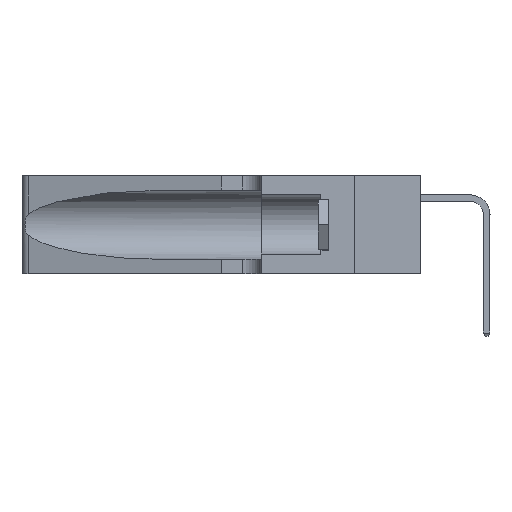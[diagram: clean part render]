
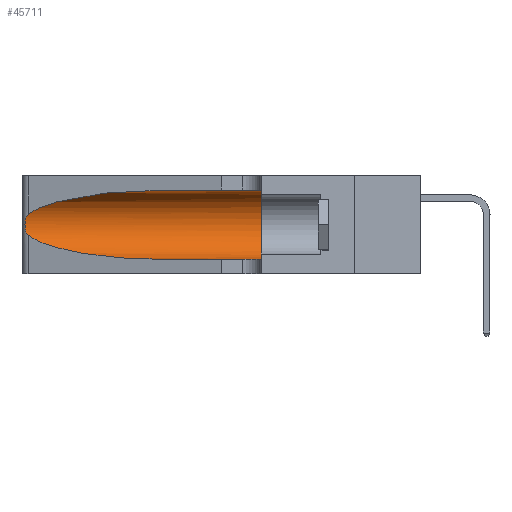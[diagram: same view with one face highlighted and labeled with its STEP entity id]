
A CAD part, left-side view. The second image highlights one B-rep face of the part: STEP entity #45711.
In plain terms, the highlighted cylindrical face has radius 3.308 mm (diameter 6.617 mm), a partial arc.
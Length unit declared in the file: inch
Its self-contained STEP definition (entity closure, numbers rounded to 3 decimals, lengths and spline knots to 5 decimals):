
#307 = DIRECTION ( 'NONE',  ( 0., 0., -1. ) ) ;
#678 = CARTESIAN_POINT ( 'NONE',  ( 0.25789, 1.23486, 0.15765 ) ) ;
#882 = EDGE_CURVE ( 'NONE', #23409, #2282, #24802, .T. ) ;
#1364 = VERTEX_POINT ( 'NONE', #19100 ) ;
#1776 =( BOUNDED_CURVE ( )  B_SPLINE_CURVE ( 3, ( #38948, #4856, #16434, #42914 ),
 .UNSPECIFIED., .F., .F. ) 
 B_SPLINE_CURVE_WITH_KNOTS ( ( 4, 4 ),
 ( 1.5708, 2.84003 ),
 .UNSPECIFIED. ) 
 CURVE ( )  GEOMETRIC_REPRESENTATION_ITEM ( )  RATIONAL_B_SPLINE_CURVE ( ( 1., 0.87, 0.87, 1. ) ) 
 REPRESENTATION_ITEM ( '' )  );
#2228 = CARTESIAN_POINT ( 'NONE',  ( 0.25487, 1.22718, 0.14631 ) ) ;
#2282 = VERTEX_POINT ( 'NONE', #2228 ) ;
#2468 = CARTESIAN_POINT ( 'NONE',  ( 0.1305, 0.72297, 0.05475 ) ) ;
#3626 = EDGE_CURVE ( 'NONE', #2282, #36121, #33569, .T. ) ;
#4567 = CARTESIAN_POINT ( 'NONE',  ( 0.25555, 1.22993, 0.14849 ) ) ;
#4856 = CARTESIAN_POINT ( 'NONE',  ( 0.18966, 0.96281, 0.31525 ) ) ;
#5522 = DIRECTION ( 'NONE',  ( 0., 1., 0. ) ) ;
#7322 = LINE ( 'NONE', #32075, #45301 ) ;
#7620 = EDGE_LOOP ( 'NONE', ( #49244, #40331, #35608, #29125, #20282, #24441 ) ) ;
#8314 = CARTESIAN_POINT ( 'NONE',  ( 0.25639, 1.23184, 0.21858 ) ) ;
#9125 = CYLINDRICAL_SURFACE ( 'NONE', #21257, 0.13025 ) ;
#9992 = EDGE_CURVE ( 'NONE', #36121, #33123, #7322, .T. ) ;
#12195 = CARTESIAN_POINT ( 'NONE',  ( 0.25787, 1.23484, 0.2124 ) ) ;
#14145 = VERTEX_POINT ( 'NONE', #47526 ) ;
#16002 = CARTESIAN_POINT ( 'NONE',  ( 0.26018, 1.23835, 0.19895 ) ) ;
#16434 = CARTESIAN_POINT ( 'NONE',  ( 0.2373, 1.15595, 0.28018 ) ) ;
#17002 = DIRECTION ( 'NONE',  ( 0., -1., 0. ) ) ;
#17243 = CARTESIAN_POINT ( 'NONE',  ( 0.1305, 0.72297, 0.05475 ) ) ;
#17751 = CARTESIAN_POINT ( 'NONE',  ( 0.2373, 1.15595, 0.08982 ) ) ;
#17806 = EDGE_CURVE ( 'NONE', #14145, #23409, #1776, .T. ) ;
#19100 = CARTESIAN_POINT ( 'NONE',  ( 0.1305, 0.35, 0.31525 ) ) ;
#19463 = CARTESIAN_POINT ( 'NONE',  ( 0.1305, 1.61858, 0.185 ) ) ;
#19827 = CARTESIAN_POINT ( 'NONE',  ( 0.26075, 1.23896, 0.178 ) ) ;
#20282 = ORIENTED_EDGE ( 'NONE', *, *, #33755, .F. ) ;
#20461 = FACE_OUTER_BOUND ( 'NONE', #7620, .T. ) ;
#21257 = AXIS2_PLACEMENT_3D ( 'NONE', #19463, #27067, #307 ) ;
#21596 = VECTOR ( 'NONE', #22932, 39.37008 ) ;
#22244 = CARTESIAN_POINT ( 'NONE',  ( 0.25487, 1.22718, 0.22369 ) ) ;
#22932 = DIRECTION ( 'NONE',  ( 0., -1., 0. ) ) ;
#23409 = VERTEX_POINT ( 'NONE', #22244 ) ;
#23631 = CARTESIAN_POINT ( 'NONE',  ( 0.25856, 1.23593, 0.16098 ) ) ;
#24441 = ORIENTED_EDGE ( 'NONE', *, *, #35800, .F. ) ;
#24802 = B_SPLINE_CURVE_WITH_KNOTS ( 'NONE', 3,
 ( #34852, #31068, #8314, #12195, #38648, #16002, #42487, #19827, #46276, #23631, #678, #27421, #4567, #31230 ),
 .UNSPECIFIED., .F., .F.,
 ( 4, 2, 2, 2, 2, 2, 4 ),
 ( 0., 0.00027, 0.00053, 0.00107, 0.0016, 0.00187, 0.00214 ),
 .UNSPECIFIED. ) ;
#25386 = CARTESIAN_POINT ( 'NONE',  ( 0.18966, 0.96281, 0.05475 ) ) ;
#27067 = DIRECTION ( 'NONE',  ( 0., -1., 0. ) ) ;
#27421 = CARTESIAN_POINT ( 'NONE',  ( 0.25639, 1.23186, 0.15144 ) ) ;
#28319 = CARTESIAN_POINT ( 'NONE',  ( 0.1305, 0.35, 0.185 ) ) ;
#29125 = ORIENTED_EDGE ( 'NONE', *, *, #9992, .T. ) ;
#31068 = CARTESIAN_POINT ( 'NONE',  ( 0.25555, 1.22994, 0.2215 ) ) ;
#31230 = CARTESIAN_POINT ( 'NONE',  ( 0.25487, 1.22718, 0.14631 ) ) ;
#32075 = CARTESIAN_POINT ( 'NONE',  ( 0.1305, 1.61858, 0.05475 ) ) ;
#32135 = DIRECTION ( 'NONE',  ( 0., 0., 1. ) ) ;
#32351 = CARTESIAN_POINT ( 'NONE',  ( 0.1305, 0.35, 0.05475 ) ) ;
#33123 = VERTEX_POINT ( 'NONE', #32351 ) ;
#33569 =( BOUNDED_CURVE ( )  B_SPLINE_CURVE ( 3, ( #44232, #17751, #25386, #2468 ),
 .UNSPECIFIED., .F., .T. ) 
 B_SPLINE_CURVE_WITH_KNOTS ( ( 4, 4 ),
 ( 3.44316, 4.71239 ),
 .UNSPECIFIED. ) 
 CURVE ( )  GEOMETRIC_REPRESENTATION_ITEM ( )  RATIONAL_B_SPLINE_CURVE ( ( 1., 0.87, 0.87, 1. ) ) 
 REPRESENTATION_ITEM ( '' )  );
#33755 = EDGE_CURVE ( 'NONE', #1364, #33123, #40099, .T. ) ;
#34852 = CARTESIAN_POINT ( 'NONE',  ( 0.25487, 1.22718, 0.22369 ) ) ;
#35608 = ORIENTED_EDGE ( 'NONE', *, *, #3626, .T. ) ;
#35800 = EDGE_CURVE ( 'NONE', #14145, #1364, #41735, .T. ) ;
#36121 = VERTEX_POINT ( 'NONE', #17243 ) ;
#38648 = CARTESIAN_POINT ( 'NONE',  ( 0.25854, 1.2359, 0.20912 ) ) ;
#38948 = CARTESIAN_POINT ( 'NONE',  ( 0.1305, 0.72297, 0.31525 ) ) ;
#40099 = CIRCLE ( 'NONE', #40525, 0.13025 ) ;
#40331 = ORIENTED_EDGE ( 'NONE', *, *, #882, .T. ) ;
#40525 = AXIS2_PLACEMENT_3D ( 'NONE', #28319, #5522, #32135 ) ;
#41735 = LINE ( 'NONE', #41942, #21596 ) ;
#41942 = CARTESIAN_POINT ( 'NONE',  ( 0.1305, 1.61858, 0.31525 ) ) ;
#42487 = CARTESIAN_POINT ( 'NONE',  ( 0.26075, 1.23896, 0.19203 ) ) ;
#42914 = CARTESIAN_POINT ( 'NONE',  ( 0.25487, 1.22718, 0.22369 ) ) ;
#44232 = CARTESIAN_POINT ( 'NONE',  ( 0.25487, 1.22718, 0.14631 ) ) ;
#45301 = VECTOR ( 'NONE', #17002, 39.37008 ) ;
#45711 = ADVANCED_FACE ( 'NONE', ( #20461 ), #9125, .F. ) ;
#46276 = CARTESIAN_POINT ( 'NONE',  ( 0.26017, 1.23833, 0.17102 ) ) ;
#47526 = CARTESIAN_POINT ( 'NONE',  ( 0.1305, 0.72297, 0.31525 ) ) ;
#49244 = ORIENTED_EDGE ( 'NONE', *, *, #17806, .T. ) ;
